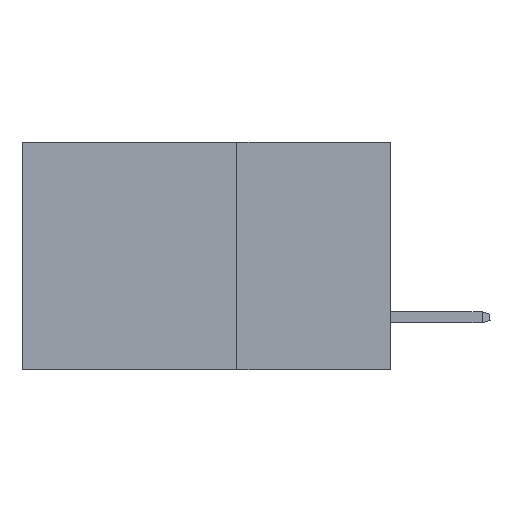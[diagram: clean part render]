
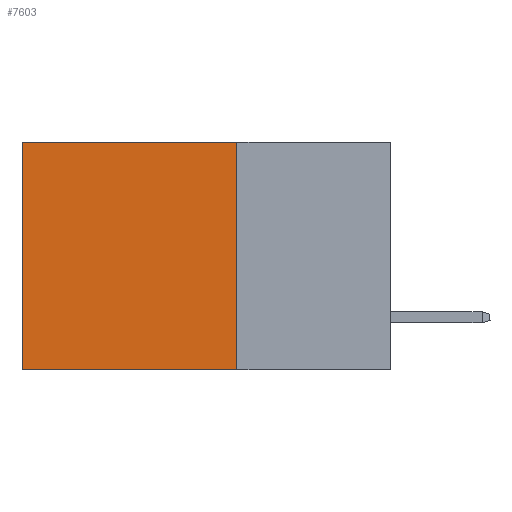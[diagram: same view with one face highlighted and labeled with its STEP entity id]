
A CAD part, left-side view. The second image highlights one B-rep face of the part: STEP entity #7603.
In plain terms, the highlighted planar face has unit normal (-1, 0, 0).
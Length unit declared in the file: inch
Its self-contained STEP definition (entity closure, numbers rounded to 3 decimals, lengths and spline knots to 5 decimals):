
#714 = VECTOR ( 'NONE', #24640, 39.37008 ) ;
#2287 = AXIS2_PLACEMENT_3D ( 'NONE', #9954, #15986, #25254 ) ;
#3145 = EDGE_CURVE ( 'NONE', #18869, #17190, #15358, .T. ) ;
#4724 = CARTESIAN_POINT ( 'NONE',  ( 0.2875, 0.25, 0. ) ) ;
#7603 = ADVANCED_FACE ( 'NONE', ( #28108 ), #37532, .F. ) ;
#9854 = CARTESIAN_POINT ( 'NONE',  ( 0.2875, 0.25, 0. ) ) ;
#9943 = VECTOR ( 'NONE', #19160, 39.37008 ) ;
#9954 = CARTESIAN_POINT ( 'NONE',  ( 0.2875, 0.25, 0. ) ) ;
#10361 = EDGE_CURVE ( 'NONE', #17190, #12655, #19355, .T. ) ;
#11319 = ORIENTED_EDGE ( 'NONE', *, *, #3145, .T. ) ;
#11383 = DIRECTION ( 'NONE',  ( 0., 0., -1. ) ) ;
#12556 = ORIENTED_EDGE ( 'NONE', *, *, #10361, .T. ) ;
#12655 = VERTEX_POINT ( 'NONE', #13255 ) ;
#13255 = CARTESIAN_POINT ( 'NONE',  ( 0.2875, 0.6, -0.37 ) ) ;
#13810 = VECTOR ( 'NONE', #11383, 39.37008 ) ;
#14276 = ORIENTED_EDGE ( 'NONE', *, *, #28954, .F. ) ;
#15358 = LINE ( 'NONE', #9854, #714 ) ;
#15904 = DIRECTION ( 'NONE',  ( 0., 1., 0. ) ) ;
#15986 = DIRECTION ( 'NONE',  ( 1., 0., 0. ) ) ;
#17190 = VERTEX_POINT ( 'NONE', #25322 ) ;
#18506 = CARTESIAN_POINT ( 'NONE',  ( 0.2875, 0.6, 0. ) ) ;
#18869 = VERTEX_POINT ( 'NONE', #32534 ) ;
#19160 = DIRECTION ( 'NONE',  ( 0., 0., -1. ) ) ;
#19355 = LINE ( 'NONE', #18506, #9943 ) ;
#19498 = CARTESIAN_POINT ( 'NONE',  ( 0.2875, 0.25, -0.37 ) ) ;
#19703 = VECTOR ( 'NONE', #15904, 39.37008 ) ;
#22042 = EDGE_CURVE ( 'NONE', #23361, #12655, #39061, .T. ) ;
#23361 = VERTEX_POINT ( 'NONE', #19498 ) ;
#24640 = DIRECTION ( 'NONE',  ( 0., 1., 0. ) ) ;
#24893 = CARTESIAN_POINT ( 'NONE',  ( 0.2875, 0.25, -0.37 ) ) ;
#25254 = DIRECTION ( 'NONE',  ( 0., 0., -1. ) ) ;
#25322 = CARTESIAN_POINT ( 'NONE',  ( 0.2875, 0.6, 0. ) ) ;
#28108 = FACE_OUTER_BOUND ( 'NONE', #28779, .T. ) ;
#28779 = EDGE_LOOP ( 'NONE', ( #12556, #30599, #14276, #11319 ) ) ;
#28954 = EDGE_CURVE ( 'NONE', #18869, #23361, #33240, .T. ) ;
#30599 = ORIENTED_EDGE ( 'NONE', *, *, #22042, .F. ) ;
#32534 = CARTESIAN_POINT ( 'NONE',  ( 0.2875, 0.25, 0. ) ) ;
#33240 = LINE ( 'NONE', #4724, #13810 ) ;
#37532 = PLANE ( 'NONE',  #2287 ) ;
#39061 = LINE ( 'NONE', #24893, #19703 ) ;
